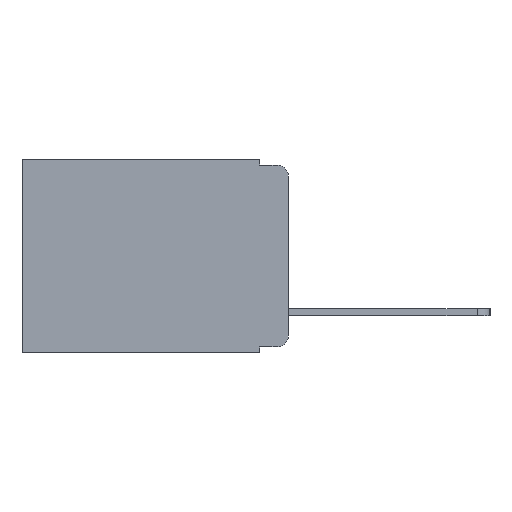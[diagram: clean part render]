
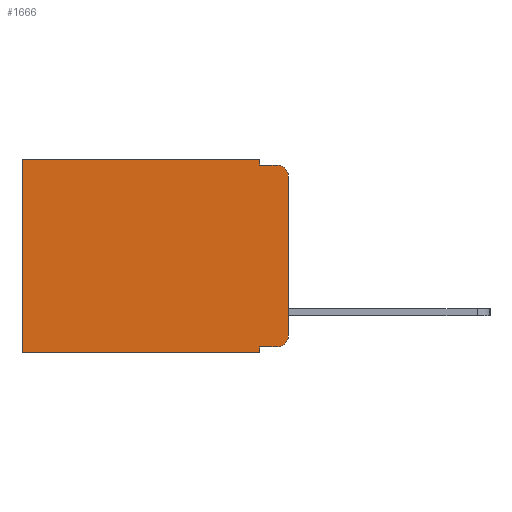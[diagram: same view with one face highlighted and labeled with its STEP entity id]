
A CAD part, left-side view. The second image highlights one B-rep face of the part: STEP entity #1666.
In plain terms, the highlighted planar face has unit normal (-1, 0, 0).
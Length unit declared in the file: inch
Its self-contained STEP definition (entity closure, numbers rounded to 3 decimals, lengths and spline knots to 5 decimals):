
#152 = ORIENTED_EDGE ( 'NONE', *, *, #8344, .F. ) ;
#171 = CARTESIAN_POINT ( 'NONE',  ( 0.298, 0.051, -0.01 ) ) ;
#212 = DIRECTION ( 'NONE',  ( 0., -1., 0. ) ) ;
#252 = LINE ( 'NONE', #612, #6791 ) ;
#393 = VERTEX_POINT ( 'NONE', #6911 ) ;
#411 = EDGE_CURVE ( 'NONE', #6571, #6398, #2396, .T. ) ;
#490 = LINE ( 'NONE', #925, #8988 ) ;
#612 = CARTESIAN_POINT ( 'NONE',  ( 0.298, 0.473, 0. ) ) ;
#873 = CARTESIAN_POINT ( 'NONE',  ( 0.298, 0., -0.313 ) ) ;
#925 = CARTESIAN_POINT ( 'NONE',  ( 0.298, 0.051, 0. ) ) ;
#976 = AXIS2_PLACEMENT_3D ( 'NONE', #6334, #1232, #7118 ) ;
#978 = DIRECTION ( 'NONE',  ( -1., 0., 0. ) ) ;
#1186 = ORIENTED_EDGE ( 'NONE', *, *, #4299, .T. ) ;
#1232 = DIRECTION ( 'NONE',  ( -1., 0., 0. ) ) ;
#1399 = VERTEX_POINT ( 'NONE', #3648 ) ;
#1571 = LINE ( 'NONE', #6746, #7683 ) ;
#1666 = ADVANCED_FACE ( 'NONE', ( #5707 ), #4139, .F. ) ;
#1734 = DIRECTION ( 'NONE',  ( 0., 0., -1. ) ) ;
#1837 = EDGE_CURVE ( 'NONE', #8833, #1399, #9875, .T. ) ;
#1875 = VERTEX_POINT ( 'NONE', #2751 ) ;
#1959 = CIRCLE ( 'NONE', #3763, 0.02 ) ;
#2055 = CARTESIAN_POINT ( 'NONE',  ( 0.298, 0.02, -0.01 ) ) ;
#2125 = VECTOR ( 'NONE', #9689, 39.37008 ) ;
#2177 = ORIENTED_EDGE ( 'NONE', *, *, #9928, .T. ) ;
#2294 = CARTESIAN_POINT ( 'NONE',  ( 0.298, 0.051, 0. ) ) ;
#2396 = LINE ( 'NONE', #6641, #2125 ) ;
#2483 = ORIENTED_EDGE ( 'NONE', *, *, #1837, .F. ) ;
#2519 = CIRCLE ( 'NONE', #976, 0.02 ) ;
#2751 = CARTESIAN_POINT ( 'NONE',  ( 0.298, 0., -0.03 ) ) ;
#2867 = DIRECTION ( 'NONE',  ( 0., 1., 0. ) ) ;
#3310 = ORIENTED_EDGE ( 'NONE', *, *, #10595, .F. ) ;
#3318 = DIRECTION ( 'NONE',  ( 0., 0., -1. ) ) ;
#3542 = CARTESIAN_POINT ( 'NONE',  ( 0.298, 0.051, -0.333 ) ) ;
#3632 = VECTOR ( 'NONE', #6989, 39.37008 ) ;
#3648 = CARTESIAN_POINT ( 'NONE',  ( 0.298, 0.051, -0.01 ) ) ;
#3763 = AXIS2_PLACEMENT_3D ( 'NONE', #6125, #978, #6885 ) ;
#3801 = ORIENTED_EDGE ( 'NONE', *, *, #8026, .F. ) ;
#3839 = ORIENTED_EDGE ( 'NONE', *, *, #5851, .F. ) ;
#3985 = DIRECTION ( 'NONE',  ( 0., 1., 0. ) ) ;
#3990 = CARTESIAN_POINT ( 'NONE',  ( 0.298, 0., 0. ) ) ;
#4081 = ORIENTED_EDGE ( 'NONE', *, *, #411, .T. ) ;
#4139 = PLANE ( 'NONE',  #8624 ) ;
#4166 = VERTEX_POINT ( 'NONE', #9433 ) ;
#4181 = ORIENTED_EDGE ( 'NONE', *, *, #9372, .T. ) ;
#4199 = DIRECTION ( 'NONE',  ( 1., 0., 0. ) ) ;
#4299 = EDGE_CURVE ( 'NONE', #8833, #393, #8901, .T. ) ;
#4351 = ORIENTED_EDGE ( 'NONE', *, *, #9627, .T. ) ;
#4601 = VERTEX_POINT ( 'NONE', #4973 ) ;
#4973 = CARTESIAN_POINT ( 'NONE',  ( 0.298, 0.051, -0.343 ) ) ;
#5274 = VERTEX_POINT ( 'NONE', #873 ) ;
#5707 = FACE_OUTER_BOUND ( 'NONE', #8449, .T. ) ;
#5798 = DIRECTION ( 'NONE',  ( 0., 0., -1. ) ) ;
#5851 = EDGE_CURVE ( 'NONE', #6571, #4601, #490, .T. ) ;
#6125 = CARTESIAN_POINT ( 'NONE',  ( 0.298, 0.02, -0.03 ) ) ;
#6331 = VERTEX_POINT ( 'NONE', #2055 ) ;
#6334 = CARTESIAN_POINT ( 'NONE',  ( 0.298, 0.02, -0.313 ) ) ;
#6348 = CARTESIAN_POINT ( 'NONE',  ( 0.298, 0., 0. ) ) ;
#6398 = VERTEX_POINT ( 'NONE', #7914 ) ;
#6465 = VECTOR ( 'NONE', #3985, 39.37008 ) ;
#6571 = VERTEX_POINT ( 'NONE', #3542 ) ;
#6641 = CARTESIAN_POINT ( 'NONE',  ( 0.298, 0.051, -0.333 ) ) ;
#6746 = CARTESIAN_POINT ( 'NONE',  ( 0.298, 0., 0. ) ) ;
#6791 = VECTOR ( 'NONE', #3318, 39.37008 ) ;
#6882 = VECTOR ( 'NONE', #2867, 39.37008 ) ;
#6885 = DIRECTION ( 'NONE',  ( 0., 0., -1. ) ) ;
#6911 = CARTESIAN_POINT ( 'NONE',  ( 0.298, 0.473, 0. ) ) ;
#6989 = DIRECTION ( 'NONE',  ( 0., 0., -1. ) ) ;
#7118 = DIRECTION ( 'NONE',  ( 0., 0., -1. ) ) ;
#7456 = CARTESIAN_POINT ( 'NONE',  ( 0.298, 0.051, 0. ) ) ;
#7683 = VECTOR ( 'NONE', #1734, 39.37008 ) ;
#7914 = CARTESIAN_POINT ( 'NONE',  ( 0.298, 0.02, -0.333 ) ) ;
#8026 = EDGE_CURVE ( 'NONE', #4601, #4166, #10486, .T. ) ;
#8315 = VECTOR ( 'NONE', #212, 39.37008 ) ;
#8344 = EDGE_CURVE ( 'NONE', #1875, #5274, #1571, .T. ) ;
#8449 = EDGE_LOOP ( 'NONE', ( #152, #2177, #3310, #2483, #1186, #4351, #3801, #3839, #4081, #4181 ) ) ;
#8463 = DIRECTION ( 'NONE',  ( 0., 0., -1. ) ) ;
#8624 = AXIS2_PLACEMENT_3D ( 'NONE', #3990, #4199, #5798 ) ;
#8676 = CARTESIAN_POINT ( 'NONE',  ( 0.298, 0., -0.343 ) ) ;
#8833 = VERTEX_POINT ( 'NONE', #2294 ) ;
#8901 = LINE ( 'NONE', #6348, #6882 ) ;
#8988 = VECTOR ( 'NONE', #8463, 39.37008 ) ;
#9372 = EDGE_CURVE ( 'NONE', #6398, #5274, #2519, .T. ) ;
#9433 = CARTESIAN_POINT ( 'NONE',  ( 0.298, 0.473, -0.343 ) ) ;
#9627 = EDGE_CURVE ( 'NONE', #393, #4166, #252, .T. ) ;
#9689 = DIRECTION ( 'NONE',  ( 0., -1., 0. ) ) ;
#9875 = LINE ( 'NONE', #7456, #3632 ) ;
#9928 = EDGE_CURVE ( 'NONE', #1875, #6331, #1959, .T. ) ;
#10327 = LINE ( 'NONE', #171, #8315 ) ;
#10486 = LINE ( 'NONE', #8676, #6465 ) ;
#10595 = EDGE_CURVE ( 'NONE', #1399, #6331, #10327, .T. ) ;
